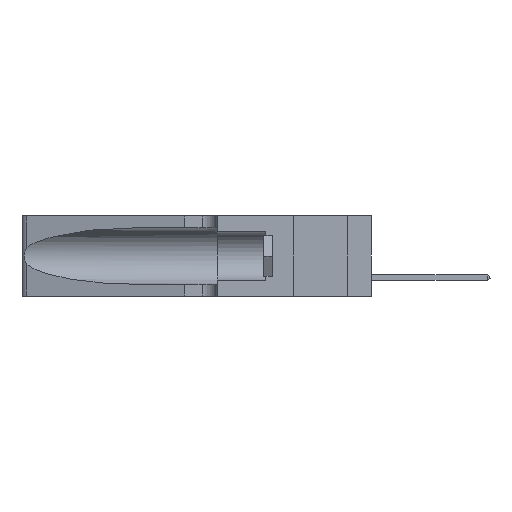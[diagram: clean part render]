
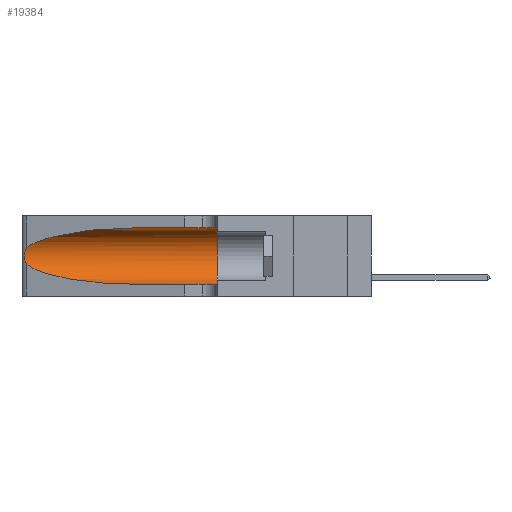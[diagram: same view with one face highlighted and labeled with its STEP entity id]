
A CAD part, left-side view. The second image highlights one B-rep face of the part: STEP entity #19384.
In plain terms, the highlighted cylindrical face has radius 3.308 mm (diameter 6.617 mm), a partial arc.
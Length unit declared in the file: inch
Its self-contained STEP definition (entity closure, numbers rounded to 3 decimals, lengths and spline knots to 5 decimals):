
#4 = VERTEX_POINT ( 'NONE', #13703 ) ;
#594 = CARTESIAN_POINT ( 'NONE',  ( 0.26017, 1.23833, 0.17102 ) ) ;
#625 = VERTEX_POINT ( 'NONE', #23246 ) ;
#906 = CARTESIAN_POINT ( 'NONE',  ( 0.1305, 1.61858, 0.05475 ) ) ;
#1533 = CARTESIAN_POINT ( 'NONE',  ( 0.25487, 1.22718, 0.22369 ) ) ;
#1687 = CARTESIAN_POINT ( 'NONE',  ( 0.25487, 1.22718, 0.14631 ) ) ;
#2722 = VECTOR ( 'NONE', #22945, 39.37008 ) ;
#2807 = EDGE_LOOP ( 'NONE', ( #28600, #3166, #7500, #32898, #4752, #22539 ) ) ;
#2926 = VERTEX_POINT ( 'NONE', #18860 ) ;
#3105 = CARTESIAN_POINT ( 'NONE',  ( 0.25487, 1.22718, 0.14631 ) ) ;
#3166 = ORIENTED_EDGE ( 'NONE', *, *, #25588, .T. ) ;
#3218 = CARTESIAN_POINT ( 'NONE',  ( 0.25487, 1.22718, 0.22369 ) ) ;
#4676 = CARTESIAN_POINT ( 'NONE',  ( 0.2373, 1.15595, 0.08982 ) ) ;
#4752 = ORIENTED_EDGE ( 'NONE', *, *, #17732, .F. ) ;
#5894 = CARTESIAN_POINT ( 'NONE',  ( 0.25555, 1.22993, 0.14849 ) ) ;
#5938 = AXIS2_PLACEMENT_3D ( 'NONE', #8288, #32125, #21614 ) ;
#6516 = CARTESIAN_POINT ( 'NONE',  ( 0.1305, 0.35, 0.31525 ) ) ;
#6822 = CARTESIAN_POINT ( 'NONE',  ( 0.25854, 1.2359, 0.20912 ) ) ;
#7500 = ORIENTED_EDGE ( 'NONE', *, *, #17171, .T. ) ;
#7644 = CARTESIAN_POINT ( 'NONE',  ( 0.26018, 1.23835, 0.19895 ) ) ;
#8288 = CARTESIAN_POINT ( 'NONE',  ( 0.1305, 0.35, 0.185 ) ) ;
#9036 = CARTESIAN_POINT ( 'NONE',  ( 0.2373, 1.15595, 0.28018 ) ) ;
#9145 = B_SPLINE_CURVE_WITH_KNOTS ( 'NONE', 3,
 ( #3218, #20542, #13493, #29700, #6822, #7644, #10471, #23626, #594, #26295, #28956, #15902, #5894, #3105 ),
 .UNSPECIFIED., .F., .F.,
 ( 4, 2, 2, 2, 2, 2, 4 ),
 ( 0., 0.00027, 0.00053, 0.00107, 0.0016, 0.00187, 0.00214 ),
 .UNSPECIFIED. ) ;
#9927 = DIRECTION ( 'NONE',  ( 0., 0., -1. ) ) ;
#10228 = CARTESIAN_POINT ( 'NONE',  ( 0.1305, 0.72297, 0.05475 ) ) ;
#10471 = CARTESIAN_POINT ( 'NONE',  ( 0.26075, 1.23896, 0.19203 ) ) ;
#11153 = AXIS2_PLACEMENT_3D ( 'NONE', #12651, #17911, #9927 ) ;
#11569 = CARTESIAN_POINT ( 'NONE',  ( 0.1305, 0.72297, 0.05475 ) ) ;
#12582 = VERTEX_POINT ( 'NONE', #11569 ) ;
#12632 = VERTEX_POINT ( 'NONE', #6516 ) ;
#12651 = CARTESIAN_POINT ( 'NONE',  ( 0.1305, 1.61858, 0.185 ) ) ;
#12930 = LINE ( 'NONE', #906, #2722 ) ;
#13493 = CARTESIAN_POINT ( 'NONE',  ( 0.25639, 1.23184, 0.21858 ) ) ;
#13703 = CARTESIAN_POINT ( 'NONE',  ( 0.25487, 1.22718, 0.22369 ) ) ;
#13842 = VERTEX_POINT ( 'NONE', #1687 ) ;
#14161 = CARTESIAN_POINT ( 'NONE',  ( 0.1305, 0.72297, 0.31525 ) ) ;
#15414 = LINE ( 'NONE', #19036, #26431 ) ;
#15902 = CARTESIAN_POINT ( 'NONE',  ( 0.25639, 1.23186, 0.15144 ) ) ;
#16871 = CYLINDRICAL_SURFACE ( 'NONE', #11153, 0.13025 ) ;
#17171 = EDGE_CURVE ( 'NONE', #13842, #12582, #17730, .T. ) ;
#17307 = EDGE_CURVE ( 'NONE', #2926, #12632, #15414, .T. ) ;
#17626 = EDGE_CURVE ( 'NONE', #12582, #625, #12930, .T. ) ;
#17730 =( BOUNDED_CURVE ( )  B_SPLINE_CURVE ( 3, ( #25143, #4676, #23388, #10228 ),
 .UNSPECIFIED., .F., .F. ) 
 B_SPLINE_CURVE_WITH_KNOTS ( ( 4, 4 ),
 ( 3.44316, 4.71239 ),
 .UNSPECIFIED. ) 
 CURVE ( )  GEOMETRIC_REPRESENTATION_ITEM ( )  RATIONAL_B_SPLINE_CURVE ( ( 1., 0.87, 0.87, 1. ) ) 
 REPRESENTATION_ITEM ( '' )  );
#17732 = EDGE_CURVE ( 'NONE', #12632, #625, #20270, .T. ) ;
#17911 = DIRECTION ( 'NONE',  ( 0., -1., 0. ) ) ;
#18860 = CARTESIAN_POINT ( 'NONE',  ( 0.1305, 0.72297, 0.31525 ) ) ;
#19036 = CARTESIAN_POINT ( 'NONE',  ( 0.1305, 1.61858, 0.31525 ) ) ;
#19384 = ADVANCED_FACE ( 'NONE', ( #30016 ), #16871, .F. ) ;
#20270 = CIRCLE ( 'NONE', #5938, 0.13025 ) ;
#20542 = CARTESIAN_POINT ( 'NONE',  ( 0.25555, 1.22994, 0.2215 ) ) ;
#21614 = DIRECTION ( 'NONE',  ( 0., 0., 1. ) ) ;
#22334 =( BOUNDED_CURVE ( )  B_SPLINE_CURVE ( 3, ( #14161, #24724, #9036, #1533 ),
 .UNSPECIFIED., .F., .F. ) 
 B_SPLINE_CURVE_WITH_KNOTS ( ( 4, 4 ),
 ( 1.5708, 2.84003 ),
 .UNSPECIFIED. ) 
 CURVE ( )  GEOMETRIC_REPRESENTATION_ITEM ( )  RATIONAL_B_SPLINE_CURVE ( ( 1., 0.87, 0.87, 1. ) ) 
 REPRESENTATION_ITEM ( '' )  );
#22539 = ORIENTED_EDGE ( 'NONE', *, *, #17307, .F. ) ;
#22945 = DIRECTION ( 'NONE',  ( 0., -1., 0. ) ) ;
#23246 = CARTESIAN_POINT ( 'NONE',  ( 0.1305, 0.35, 0.05475 ) ) ;
#23388 = CARTESIAN_POINT ( 'NONE',  ( 0.18966, 0.96281, 0.05475 ) ) ;
#23626 = CARTESIAN_POINT ( 'NONE',  ( 0.26075, 1.23896, 0.178 ) ) ;
#24724 = CARTESIAN_POINT ( 'NONE',  ( 0.18966, 0.96281, 0.31525 ) ) ;
#25143 = CARTESIAN_POINT ( 'NONE',  ( 0.25487, 1.22718, 0.14631 ) ) ;
#25588 = EDGE_CURVE ( 'NONE', #4, #13842, #9145, .T. ) ;
#26295 = CARTESIAN_POINT ( 'NONE',  ( 0.25856, 1.23593, 0.16098 ) ) ;
#26431 = VECTOR ( 'NONE', #30191, 39.37008 ) ;
#28600 = ORIENTED_EDGE ( 'NONE', *, *, #32765, .T. ) ;
#28956 = CARTESIAN_POINT ( 'NONE',  ( 0.25789, 1.23486, 0.15765 ) ) ;
#29700 = CARTESIAN_POINT ( 'NONE',  ( 0.25787, 1.23484, 0.2124 ) ) ;
#30016 = FACE_OUTER_BOUND ( 'NONE', #2807, .T. ) ;
#30191 = DIRECTION ( 'NONE',  ( 0., -1., 0. ) ) ;
#32125 = DIRECTION ( 'NONE',  ( 0., 1., 0. ) ) ;
#32765 = EDGE_CURVE ( 'NONE', #2926, #4, #22334, .T. ) ;
#32898 = ORIENTED_EDGE ( 'NONE', *, *, #17626, .T. ) ;
